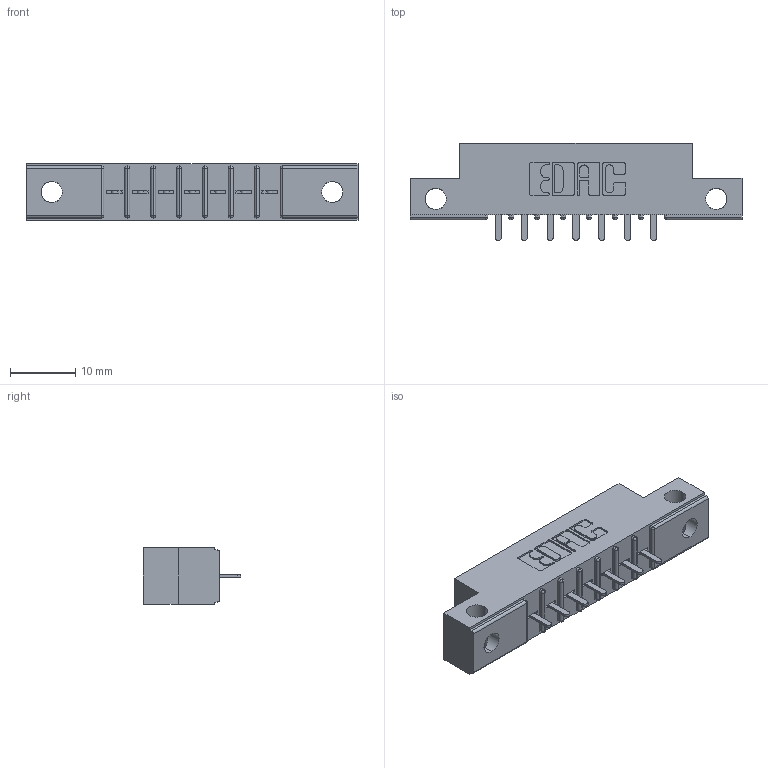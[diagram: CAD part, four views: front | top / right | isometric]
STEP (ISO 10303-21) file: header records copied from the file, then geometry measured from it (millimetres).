
FILE_DESCRIPTION (( 'STEP AP203' ), '1' );
FILE_NAME ('356-007-521-112.STEP', '2020-09-20T21:49:19', ( '' ), ( '' ), 'SwSTEP 2.0', 'SolidWorks 2020', '' );
FILE_SCHEMA (( 'CONFIG_CONTROL_DESIGN' ));
Length unit declared in the file: inch
Products named in the file (3): 306-290-001_121; 356-007-521-112; 306 Part_.128 Dia
Assembly tree (8 placements, depth 2):
  356-007-521-112
    306 Part_.128 Dia
    306-290-001_121  x7
Bounding box: 50.75 x 14.88 x 8.71 mm (x, y, z)
Volume: 3256.2 mm3; surface area: 4247.3 mm2
Topology: 8 solids, 8 shells, 618 faces, 1731 edges, 1110 vertices
Faces by surface type: plane 397, cylinder 193, sphere 28
Entity records: 11424 total; most frequent: CARTESIAN_POINT 1960, ORIENTED_EDGE 1894, DIRECTION 1875, EDGE_CURVE 947, LINE 705, VECTOR 705, VERTEX_POINT 606, AXIS2_PLACEMENT_3D 585
